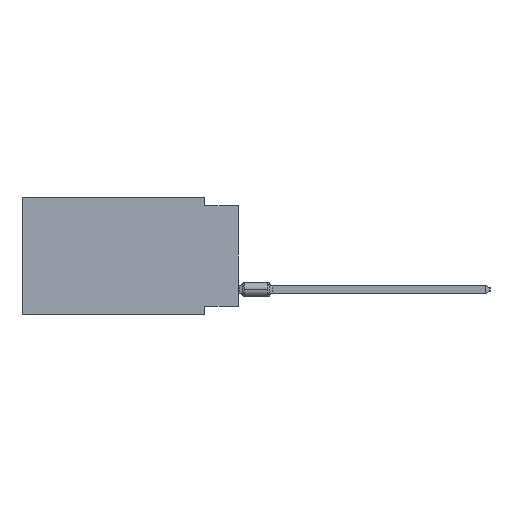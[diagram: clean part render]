
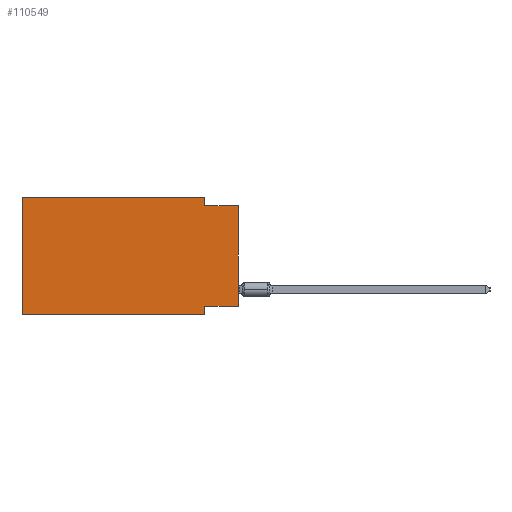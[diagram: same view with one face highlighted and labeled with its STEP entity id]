
A CAD part, left-side view. The second image highlights one B-rep face of the part: STEP entity #110549.
In plain terms, the highlighted planar face has unit normal (-1, 0, 0).
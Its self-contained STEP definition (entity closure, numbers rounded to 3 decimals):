
#1728 = VECTOR ( 'NONE', #79934, 1000. ) ;
#4131 = EDGE_CURVE ( 'NONE', #114075, #96944, #4563, .T. ) ;
#4563 = LINE ( 'NONE', #43767, #1728 ) ;
#5135 = DIRECTION ( 'NONE',  ( 0., 0., -1. ) ) ;
#5728 = LINE ( 'NONE', #52183, #56794 ) ;
#6776 = EDGE_CURVE ( 'NONE', #106212, #114075, #119324, .T. ) ;
#7038 = DIRECTION ( 'NONE',  ( 0., 0., 1. ) ) ;
#7776 = LINE ( 'NONE', #63250, #58302 ) ;
#8258 = CARTESIAN_POINT ( 'NONE',  ( 0., 16.383, 0. ) ) ;
#17287 = CARTESIAN_POINT ( 'NONE',  ( 0., 16.383, 0. ) ) ;
#18177 = DIRECTION ( 'NONE',  ( 0., 0., -1. ) ) ;
#20648 = CARTESIAN_POINT ( 'NONE',  ( 0., 0., -0.635 ) ) ;
#21254 = ORIENTED_EDGE ( 'NONE', *, *, #51611, .F. ) ;
#22165 = CARTESIAN_POINT ( 'NONE',  ( 0., 2.54, 0. ) ) ;
#25295 = VERTEX_POINT ( 'NONE', #62116 ) ;
#31649 = LINE ( 'NONE', #107026, #58378 ) ;
#33758 = VERTEX_POINT ( 'NONE', #111238 ) ;
#33878 = CARTESIAN_POINT ( 'NONE',  ( 0., 16.383, -8.89 ) ) ;
#34217 = CARTESIAN_POINT ( 'NONE',  ( 0., 0., -8.255 ) ) ;
#43330 = ORIENTED_EDGE ( 'NONE', *, *, #64013, .T. ) ;
#43767 = CARTESIAN_POINT ( 'NONE',  ( 0., 0., -0.635 ) ) ;
#48123 = VECTOR ( 'NONE', #7038, 1000. ) ;
#50233 = EDGE_CURVE ( 'NONE', #33758, #25295, #5728, .T. ) ;
#51611 = EDGE_CURVE ( 'NONE', #111275, #106212, #7776, .T. ) ;
#51868 = EDGE_CURVE ( 'NONE', #98803, #96944, #31649, .T. ) ;
#52183 = CARTESIAN_POINT ( 'NONE',  ( 0., 2.54, -8.89 ) ) ;
#53108 = VERTEX_POINT ( 'NONE', #61358 ) ;
#54594 = ORIENTED_EDGE ( 'NONE', *, *, #72714, .F. ) ;
#55412 = DIRECTION ( 'NONE',  ( 0., -1., 0. ) ) ;
#56794 = VECTOR ( 'NONE', #5135, 1000. ) ;
#58302 = VECTOR ( 'NONE', #93828, 1000. ) ;
#58378 = VECTOR ( 'NONE', #61778, 1000. ) ;
#61358 = CARTESIAN_POINT ( 'NONE',  ( 0., 16.383, -8.89 ) ) ;
#61778 = DIRECTION ( 'NONE',  ( 0., 0., 1. ) ) ;
#62116 = CARTESIAN_POINT ( 'NONE',  ( 0., 2.54, -8.89 ) ) ;
#62325 = EDGE_LOOP ( 'NONE', ( #94204, #99669, #116662, #21254, #54594, #43330, #104222, #89170 ) ) ;
#63250 = CARTESIAN_POINT ( 'NONE',  ( 0., 16.383, 0. ) ) ;
#64013 = EDGE_CURVE ( 'NONE', #53108, #25295, #117120, .T. ) ;
#72487 = PLANE ( 'NONE',  #96152 ) ;
#72714 = EDGE_CURVE ( 'NONE', #53108, #111275, #99930, .T. ) ;
#74269 = CARTESIAN_POINT ( 'NONE',  ( 0., 16.383, 0. ) ) ;
#79049 = VECTOR ( 'NONE', #92155, 1000. ) ;
#79934 = DIRECTION ( 'NONE',  ( 0., -1., 0. ) ) ;
#83884 = DIRECTION ( 'NONE',  ( 0., 1., 0. ) ) ;
#86839 = VECTOR ( 'NONE', #83884, 1000. ) ;
#86992 = CARTESIAN_POINT ( 'NONE',  ( 0., 2.54, -0.635 ) ) ;
#89170 = ORIENTED_EDGE ( 'NONE', *, *, #114346, .F. ) ;
#91558 = CARTESIAN_POINT ( 'NONE',  ( 0., 2.54, 0. ) ) ;
#91782 = DIRECTION ( 'NONE',  ( 1., 0., 0. ) ) ;
#92155 = DIRECTION ( 'NONE',  ( 0., 0., -1. ) ) ;
#93828 = DIRECTION ( 'NONE',  ( 0., -1., 0. ) ) ;
#94204 = ORIENTED_EDGE ( 'NONE', *, *, #51868, .T. ) ;
#95133 = VECTOR ( 'NONE', #55412, 1000. ) ;
#96152 = AXIS2_PLACEMENT_3D ( 'NONE', #74269, #91782, #18177 ) ;
#96944 = VERTEX_POINT ( 'NONE', #20648 ) ;
#98803 = VERTEX_POINT ( 'NONE', #34217 ) ;
#99669 = ORIENTED_EDGE ( 'NONE', *, *, #4131, .F. ) ;
#99930 = LINE ( 'NONE', #17287, #48123 ) ;
#101432 = FACE_OUTER_BOUND ( 'NONE', #62325, .T. ) ;
#104222 = ORIENTED_EDGE ( 'NONE', *, *, #50233, .F. ) ;
#106212 = VERTEX_POINT ( 'NONE', #22165 ) ;
#107026 = CARTESIAN_POINT ( 'NONE',  ( 0., 0., 0. ) ) ;
#110549 = ADVANCED_FACE ( 'NONE', ( #101432 ), #72487, .F. ) ;
#111037 = LINE ( 'NONE', #118906, #86839 ) ;
#111238 = CARTESIAN_POINT ( 'NONE',  ( 0., 2.54, -8.255 ) ) ;
#111275 = VERTEX_POINT ( 'NONE', #8258 ) ;
#114075 = VERTEX_POINT ( 'NONE', #86992 ) ;
#114346 = EDGE_CURVE ( 'NONE', #98803, #33758, #111037, .T. ) ;
#116662 = ORIENTED_EDGE ( 'NONE', *, *, #6776, .F. ) ;
#117120 = LINE ( 'NONE', #33878, #95133 ) ;
#118906 = CARTESIAN_POINT ( 'NONE',  ( 0., 0., -8.255 ) ) ;
#119324 = LINE ( 'NONE', #91558, #79049 ) ;
